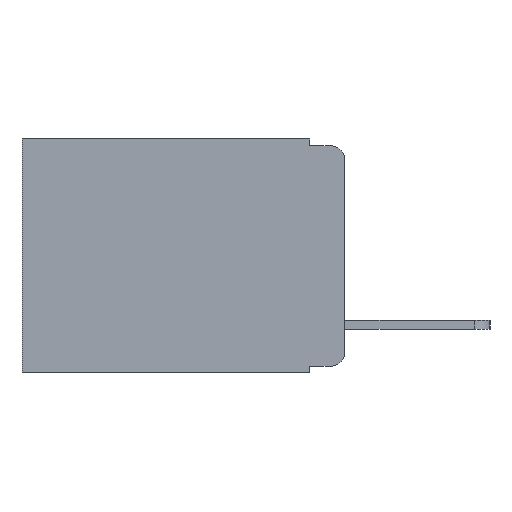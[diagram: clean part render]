
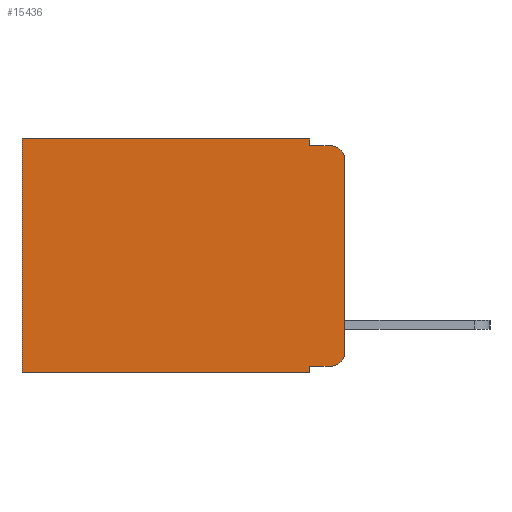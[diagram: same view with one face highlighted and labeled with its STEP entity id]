
A CAD part, left-side view. The second image highlights one B-rep face of the part: STEP entity #15436.
In plain terms, the highlighted planar face has unit normal (-1, 0, 0).
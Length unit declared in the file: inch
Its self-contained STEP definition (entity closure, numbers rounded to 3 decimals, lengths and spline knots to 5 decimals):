
#236 = VERTEX_POINT ( 'NONE', #16621 ) ;
#993 = LINE ( 'NONE', #10295, #9235 ) ;
#1005 = DIRECTION ( 'NONE',  ( 0., 0., -1. ) ) ;
#1206 = DIRECTION ( 'NONE',  ( 0., -1., 0. ) ) ;
#1287 = DIRECTION ( 'NONE',  ( 1., 0., 0. ) ) ;
#1305 = DIRECTION ( 'NONE',  ( 0., 0., -1. ) ) ;
#1357 = EDGE_CURVE ( 'NONE', #7541, #14033, #16815, .T. ) ;
#2046 = EDGE_CURVE ( 'NONE', #14033, #3212, #6258, .T. ) ;
#2086 = EDGE_CURVE ( 'NONE', #3102, #19739, #12931, .T. ) ;
#2425 = VECTOR ( 'NONE', #2680, 39.37008 ) ;
#2680 = DIRECTION ( 'NONE',  ( 0., 0., -1. ) ) ;
#3102 = VERTEX_POINT ( 'NONE', #17241 ) ;
#3212 = VERTEX_POINT ( 'NONE', #16405 ) ;
#3253 = EDGE_CURVE ( 'NONE', #3102, #3212, #6705, .T. ) ;
#3573 = CARTESIAN_POINT ( 'NONE',  ( 0.298, 0.051, 0. ) ) ;
#3631 = DIRECTION ( 'NONE',  ( 0., 0., -1. ) ) ;
#3826 = VECTOR ( 'NONE', #18319, 39.37008 ) ;
#4764 = AXIS2_PLACEMENT_3D ( 'NONE', #7548, #15278, #1305 ) ;
#4792 = FACE_OUTER_BOUND ( 'NONE', #6473, .T. ) ;
#5456 = DIRECTION ( 'NONE',  ( 0., 0., -1. ) ) ;
#5752 = EDGE_CURVE ( 'NONE', #8957, #12143, #12191, .T. ) ;
#6258 = CIRCLE ( 'NONE', #4764, 0.02 ) ;
#6374 = CARTESIAN_POINT ( 'NONE',  ( 0.298, 0., 0. ) ) ;
#6411 = CARTESIAN_POINT ( 'NONE',  ( 0.298, 0.051, -0.333 ) ) ;
#6473 = EDGE_LOOP ( 'NONE', ( #7782, #7914, #7974, #8050, #8208, #8368, #8436, #8619, #8649, #8804 ) ) ;
#6705 = LINE ( 'NONE', #15586, #9782 ) ;
#7341 = VECTOR ( 'NONE', #1206, 39.37008 ) ;
#7415 = EDGE_CURVE ( 'NONE', #236, #14213, #993, .T. ) ;
#7541 = VERTEX_POINT ( 'NONE', #6411 ) ;
#7548 = CARTESIAN_POINT ( 'NONE',  ( 0.298, 0.02, -0.313 ) ) ;
#7652 = EDGE_CURVE ( 'NONE', #7541, #8957, #10917, .T. ) ;
#7723 = CARTESIAN_POINT ( 'NONE',  ( 0.298, 0.051, -0.343 ) ) ;
#7782 = ORIENTED_EDGE ( 'NONE', *, *, #3253, .F. ) ;
#7914 = ORIENTED_EDGE ( 'NONE', *, *, #2086, .T. ) ;
#7974 = ORIENTED_EDGE ( 'NONE', *, *, #18223, .F. ) ;
#8050 = ORIENTED_EDGE ( 'NONE', *, *, #13415, .F. ) ;
#8208 = ORIENTED_EDGE ( 'NONE', *, *, #7415, .T. ) ;
#8368 = ORIENTED_EDGE ( 'NONE', *, *, #17822, .T. ) ;
#8423 = CARTESIAN_POINT ( 'NONE',  ( 0.298, 0.473, 0. ) ) ;
#8436 = ORIENTED_EDGE ( 'NONE', *, *, #5752, .F. ) ;
#8619 = ORIENTED_EDGE ( 'NONE', *, *, #7652, .F. ) ;
#8649 = ORIENTED_EDGE ( 'NONE', *, *, #1357, .T. ) ;
#8804 = ORIENTED_EDGE ( 'NONE', *, *, #2046, .T. ) ;
#8957 = VERTEX_POINT ( 'NONE', #7723 ) ;
#9065 = CARTESIAN_POINT ( 'NONE',  ( 0.298, 0.02, -0.01 ) ) ;
#9096 = CARTESIAN_POINT ( 'NONE',  ( 0.298, 0.473, -0.343 ) ) ;
#9235 = VECTOR ( 'NONE', #10346, 39.37008 ) ;
#9782 = VECTOR ( 'NONE', #16188, 39.37008 ) ;
#9962 = AXIS2_PLACEMENT_3D ( 'NONE', #16297, #16073, #1005 ) ;
#10050 = DIRECTION ( 'NONE',  ( 0., -1., 0. ) ) ;
#10286 = CARTESIAN_POINT ( 'NONE',  ( 0.298, 0.051, -0.01 ) ) ;
#10295 = CARTESIAN_POINT ( 'NONE',  ( 0.298, 0., 0. ) ) ;
#10346 = DIRECTION ( 'NONE',  ( 0., 1., 0. ) ) ;
#10386 = CARTESIAN_POINT ( 'NONE',  ( 0.298, 0.051, -0.333 ) ) ;
#10460 = VECTOR ( 'NONE', #5456, 39.37008 ) ;
#10917 = LINE ( 'NONE', #3573, #2425 ) ;
#10923 = CARTESIAN_POINT ( 'NONE',  ( 0.298, 0.051, -0.01 ) ) ;
#10926 = VERTEX_POINT ( 'NONE', #10286 ) ;
#10942 = LINE ( 'NONE', #8423, #14537 ) ;
#12143 = VERTEX_POINT ( 'NONE', #9096 ) ;
#12191 = LINE ( 'NONE', #16183, #3826 ) ;
#12535 = DIRECTION ( 'NONE',  ( 0., 0., -1. ) ) ;
#12931 = CIRCLE ( 'NONE', #9962, 0.02 ) ;
#13415 = EDGE_CURVE ( 'NONE', #236, #10926, #14536, .T. ) ;
#14033 = VERTEX_POINT ( 'NONE', #15252 ) ;
#14167 = CARTESIAN_POINT ( 'NONE',  ( 0.298, 0.473, 0. ) ) ;
#14213 = VERTEX_POINT ( 'NONE', #14167 ) ;
#14536 = LINE ( 'NONE', #16149, #10460 ) ;
#14537 = VECTOR ( 'NONE', #3631, 39.37008 ) ;
#15252 = CARTESIAN_POINT ( 'NONE',  ( 0.298, 0.02, -0.333 ) ) ;
#15278 = DIRECTION ( 'NONE',  ( -1., 0., 0. ) ) ;
#15436 = ADVANCED_FACE ( 'NONE', ( #4792 ), #19900, .F. ) ;
#15586 = CARTESIAN_POINT ( 'NONE',  ( 0.298, 0., 0. ) ) ;
#16073 = DIRECTION ( 'NONE',  ( -1., 0., 0. ) ) ;
#16149 = CARTESIAN_POINT ( 'NONE',  ( 0.298, 0.051, 0. ) ) ;
#16183 = CARTESIAN_POINT ( 'NONE',  ( 0.298, 0., -0.343 ) ) ;
#16188 = DIRECTION ( 'NONE',  ( 0., 0., -1. ) ) ;
#16297 = CARTESIAN_POINT ( 'NONE',  ( 0.298, 0.02, -0.03 ) ) ;
#16405 = CARTESIAN_POINT ( 'NONE',  ( 0.298, 0., -0.313 ) ) ;
#16621 = CARTESIAN_POINT ( 'NONE',  ( 0.298, 0.051, 0. ) ) ;
#16815 = LINE ( 'NONE', #10386, #20119 ) ;
#17241 = CARTESIAN_POINT ( 'NONE',  ( 0.298, 0., -0.03 ) ) ;
#17822 = EDGE_CURVE ( 'NONE', #14213, #12143, #10942, .T. ) ;
#18223 = EDGE_CURVE ( 'NONE', #10926, #19739, #18925, .T. ) ;
#18319 = DIRECTION ( 'NONE',  ( 0., 1., 0. ) ) ;
#18925 = LINE ( 'NONE', #10923, #7341 ) ;
#19141 = AXIS2_PLACEMENT_3D ( 'NONE', #6374, #1287, #12535 ) ;
#19739 = VERTEX_POINT ( 'NONE', #9065 ) ;
#19900 = PLANE ( 'NONE',  #19141 ) ;
#20119 = VECTOR ( 'NONE', #10050, 39.37008 ) ;
